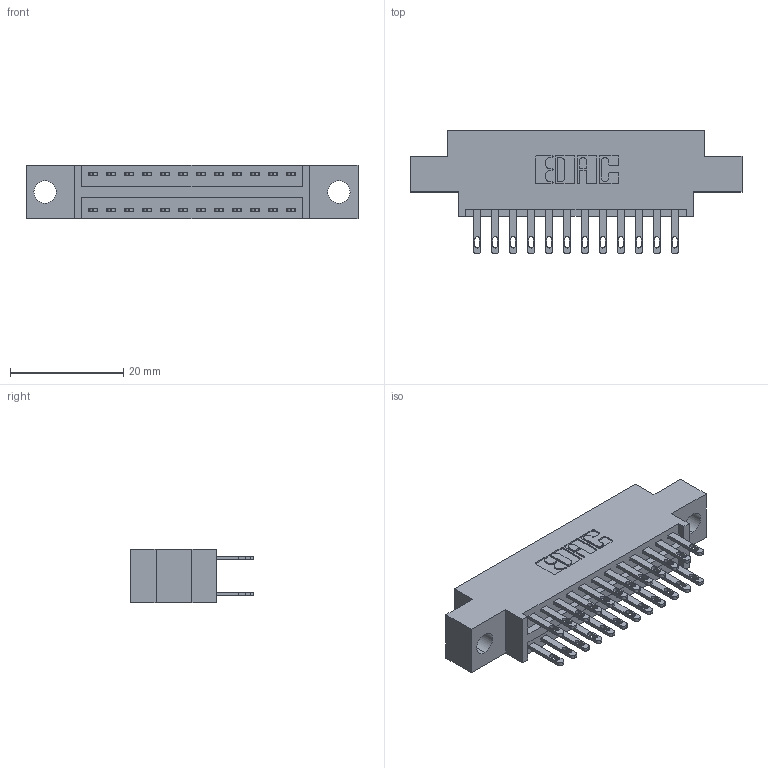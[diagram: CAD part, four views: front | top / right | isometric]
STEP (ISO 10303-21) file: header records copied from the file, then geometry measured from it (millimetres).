
FILE_DESCRIPTION (( 'STEP AP203' ), '1' );
FILE_NAME ('346-024-500-804.STEP', '2022-05-18T22:37:48', ( '' ), ( '' ), 'SwSTEP 2.0', 'SolidWorks 2020', '' );
FILE_SCHEMA (( 'CONFIG_CONTROL_DESIGN' ));
Length unit declared in the file: inch
Products named in the file (3): 346-024-500-804; 346 Part_0.170 Offset - 0.156 Dia-TH; 345-292-001_345-293-100
Assembly tree (25 placements, depth 2):
  346-024-500-804
    346 Part_0.170 Offset - 0.156 Dia-TH
    345-292-001_345-293-100  x24
Bounding box: 58.67 x 21.84 x 9.4 mm (x, y, z)
Volume: 5301.2 mm3; surface area: 7094.1 mm2
Topology: 25 solids, 25 shells, 1292 faces, 3905 edges, 2602 vertices
Faces by surface type: plane 790, cylinder 502
Entity records: 12351 total; most frequent: CARTESIAN_POINT 2082, ORIENTED_EDGE 2014, DIRECTION 1887, EDGE_CURVE 1007, LINE 823, VECTOR 823, VERTEX_POINT 670, AXIS2_PLACEMENT_3D 532
